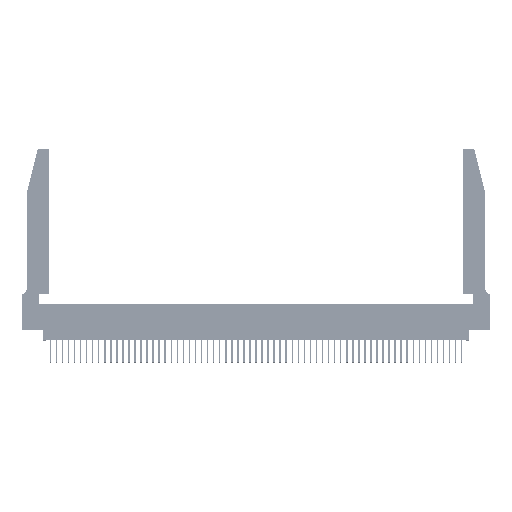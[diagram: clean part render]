
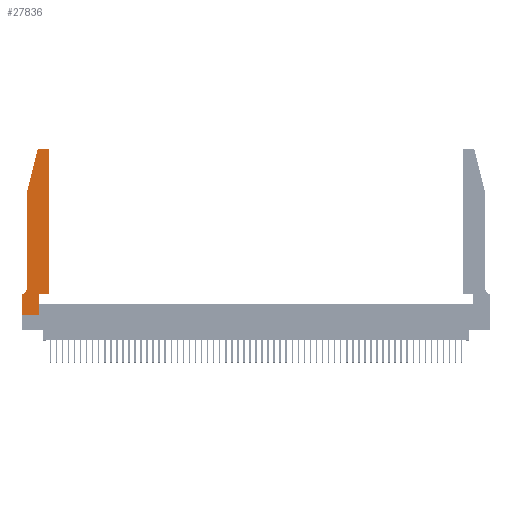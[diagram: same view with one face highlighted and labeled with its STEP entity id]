
A CAD part, top view. The second image highlights one B-rep face of the part: STEP entity #27836.
In plain terms, the highlighted planar face has unit normal (0, 0, 1).
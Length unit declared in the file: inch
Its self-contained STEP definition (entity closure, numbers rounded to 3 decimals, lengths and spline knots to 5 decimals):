
#403 = AXIS2_PLACEMENT_3D ( 'NONE', #30893, #5789, #18160 ) ;
#785 = EDGE_CURVE ( 'NONE', #35625, #1669, #9941, .T. ) ;
#947 = CARTESIAN_POINT ( 'NONE',  ( 0.284, 2.75, 0.37 ) ) ;
#1004 = ORIENTED_EDGE ( 'NONE', *, *, #785, .T. ) ;
#1669 = VERTEX_POINT ( 'NONE', #38193 ) ;
#1756 = VERTEX_POINT ( 'NONE', #46417 ) ;
#3053 = CARTESIAN_POINT ( 'NONE',  ( 0.4205, 2.72, 0.37 ) ) ;
#3824 = AXIS2_PLACEMENT_3D ( 'NONE', #3053, #15457, #7031 ) ;
#4704 = CARTESIAN_POINT ( 'NONE',  ( 0.4505, 0.35, 0.37 ) ) ;
#5002 = VERTEX_POINT ( 'NONE', #35126 ) ;
#5269 = DIRECTION ( 'NONE',  ( -1., 0., 0. ) ) ;
#5352 = ORIENTED_EDGE ( 'NONE', *, *, #52230, .T. ) ;
#5355 = VERTEX_POINT ( 'NONE', #29994 ) ;
#5673 = DIRECTION ( 'NONE',  ( -0.239, -0.971, 0. ) ) ;
#5789 = DIRECTION ( 'NONE',  ( 0., 0., 1. ) ) ;
#6862 = VECTOR ( 'NONE', #18560, 39.37008 ) ;
#7031 = DIRECTION ( 'NONE',  ( 1., 0., 0. ) ) ;
#7310 = CARTESIAN_POINT ( 'NONE',  ( 0.284, 2.72, 0.37 ) ) ;
#7510 = ORIENTED_EDGE ( 'NONE', *, *, #41520, .T. ) ;
#8234 = LINE ( 'NONE', #52009, #48363 ) ;
#9884 = VECTOR ( 'NONE', #24211, 39.37008 ) ;
#9941 = CIRCLE ( 'NONE', #3824, 0.03 ) ;
#10123 = EDGE_CURVE ( 'NONE', #1669, #36552, #8234, .T. ) ;
#11624 = DIRECTION ( 'NONE',  ( 1., 0., 0. ) ) ;
#12800 = VECTOR ( 'NONE', #5673, 39.37008 ) ;
#12887 = LINE ( 'NONE', #43791, #52960 ) ;
#13272 = VERTEX_POINT ( 'NONE', #48059 ) ;
#13618 = CARTESIAN_POINT ( 'NONE',  ( 0.0755, 2., 0.37 ) ) ;
#15457 = DIRECTION ( 'NONE',  ( 0., 0., 1. ) ) ;
#16917 = ORIENTED_EDGE ( 'NONE', *, *, #40889, .T. ) ;
#17618 = LINE ( 'NONE', #30756, #6862 ) ;
#18160 = DIRECTION ( 'NONE',  ( 1., 0., 0. ) ) ;
#18479 = CIRCLE ( 'NONE', #33254, 0.03 ) ;
#18560 = DIRECTION ( 'NONE',  ( 1., 0., 0. ) ) ;
#19590 = EDGE_CURVE ( 'NONE', #53398, #1756, #29552, .T. ) ;
#19633 = ORIENTED_EDGE ( 'NONE', *, *, #32566, .T. ) ;
#19774 = CARTESIAN_POINT ( 'NONE',  ( 0.25487, 2.72718, 0.37 ) ) ;
#20155 = CARTESIAN_POINT ( 'NONE',  ( 0.4505, 2.72, 0.37 ) ) ;
#21183 = DIRECTION ( 'NONE',  ( 1., 0., 0. ) ) ;
#22218 = DIRECTION ( 'NONE',  ( 0., -1., 0. ) ) ;
#22270 = AXIS2_PLACEMENT_3D ( 'NONE', #39279, #33523, #42101 ) ;
#24135 = ORIENTED_EDGE ( 'NONE', *, *, #49667, .T. ) ;
#24211 = DIRECTION ( 'NONE',  ( -1., 0., 0. ) ) ;
#24219 = EDGE_CURVE ( 'NONE', #32277, #42712, #30310, .T. ) ;
#25503 = EDGE_CURVE ( 'NONE', #33452, #5002, #47479, .T. ) ;
#26002 = VECTOR ( 'NONE', #43859, 39.37008 ) ;
#27297 = PLANE ( 'NONE',  #403 ) ;
#27557 = CARTESIAN_POINT ( 'NONE',  ( 0.4505, 0.35, 0.37 ) ) ;
#27836 = ADVANCED_FACE ( 'NONE', ( #40368 ), #27297, .T. ) ;
#29552 = LINE ( 'NONE', #48686, #12800 ) ;
#29994 = CARTESIAN_POINT ( 'NONE',  ( 0., 0.35, 0.37 ) ) ;
#30310 = LINE ( 'NONE', #4704, #47683 ) ;
#30756 = CARTESIAN_POINT ( 'NONE',  ( 0., 0., 0.37 ) ) ;
#30893 = CARTESIAN_POINT ( 'NONE',  ( 0., 0.35, 0.37 ) ) ;
#31427 = EDGE_CURVE ( 'NONE', #42712, #35625, #37385, .T. ) ;
#32277 = VERTEX_POINT ( 'NONE', #33971 ) ;
#32566 = EDGE_CURVE ( 'NONE', #36552, #53398, #18479, .T. ) ;
#33224 = ORIENTED_EDGE ( 'NONE', *, *, #19590, .T. ) ;
#33254 = AXIS2_PLACEMENT_3D ( 'NONE', #7310, #41540, #11624 ) ;
#33452 = VERTEX_POINT ( 'NONE', #46929 ) ;
#33523 = DIRECTION ( 'NONE',  ( 0., 0., -1. ) ) ;
#33971 = CARTESIAN_POINT ( 'NONE',  ( 0.2865, 0.35, 0.37 ) ) ;
#34423 = ORIENTED_EDGE ( 'NONE', *, *, #24219, .T. ) ;
#35126 = CARTESIAN_POINT ( 'NONE',  ( 0.0055, 0.35, 0.37 ) ) ;
#35601 = DIRECTION ( 'NONE',  ( 0., 1., 0. ) ) ;
#35625 = VERTEX_POINT ( 'NONE', #20155 ) ;
#36552 = VERTEX_POINT ( 'NONE', #947 ) ;
#37385 = LINE ( 'NONE', #27557, #26002 ) ;
#37498 = CARTESIAN_POINT ( 'NONE',  ( 0.0755, 0.35, 0.37 ) ) ;
#38193 = CARTESIAN_POINT ( 'NONE',  ( 0.4205, 2.75, 0.37 ) ) ;
#39279 = CARTESIAN_POINT ( 'NONE',  ( 0.0055, 0.42, 0.37 ) ) ;
#39545 = ORIENTED_EDGE ( 'NONE', *, *, #10123, .T. ) ;
#39900 = DIRECTION ( 'NONE',  ( 0., -1., 0. ) ) ;
#40368 = FACE_OUTER_BOUND ( 'NONE', #50018, .T. ) ;
#40889 = EDGE_CURVE ( 'NONE', #13272, #32277, #12887, .T. ) ;
#40894 = LINE ( 'NONE', #13618, #50931 ) ;
#41481 = ORIENTED_EDGE ( 'NONE', *, *, #31427, .T. ) ;
#41520 = EDGE_CURVE ( 'NONE', #1756, #33452, #40894, .T. ) ;
#41540 = DIRECTION ( 'NONE',  ( 0., 0., 1. ) ) ;
#41866 = CARTESIAN_POINT ( 'NONE',  ( 0., 0., 0.37 ) ) ;
#42101 = DIRECTION ( 'NONE',  ( -1., 0., 0. ) ) ;
#42712 = VERTEX_POINT ( 'NONE', #47709 ) ;
#43511 = VECTOR ( 'NONE', #39900, 39.37008 ) ;
#43791 = CARTESIAN_POINT ( 'NONE',  ( 0.2865, 0.35, 0.37 ) ) ;
#43859 = DIRECTION ( 'NONE',  ( 0., 1., 0. ) ) ;
#46417 = CARTESIAN_POINT ( 'NONE',  ( 0.0755, 2., 0.37 ) ) ;
#46929 = CARTESIAN_POINT ( 'NONE',  ( 0.0755, 0.42, 0.37 ) ) ;
#47384 = VERTEX_POINT ( 'NONE', #41866 ) ;
#47391 = LINE ( 'NONE', #37498, #9884 ) ;
#47479 = CIRCLE ( 'NONE', #22270, 0.07 ) ;
#47683 = VECTOR ( 'NONE', #21183, 39.37008 ) ;
#47709 = CARTESIAN_POINT ( 'NONE',  ( 0.4505, 0.35, 0.37 ) ) ;
#47957 = CARTESIAN_POINT ( 'NONE',  ( 0., 0., 0.37 ) ) ;
#48059 = CARTESIAN_POINT ( 'NONE',  ( 0.2865, 0., 0.37 ) ) ;
#48250 = EDGE_CURVE ( 'NONE', #5355, #47384, #50872, .T. ) ;
#48363 = VECTOR ( 'NONE', #5269, 39.37008 ) ;
#48686 = CARTESIAN_POINT ( 'NONE',  ( 0.0755, 2., 0.37 ) ) ;
#49667 = EDGE_CURVE ( 'NONE', #5002, #5355, #47391, .T. ) ;
#50018 = EDGE_LOOP ( 'NONE', ( #39545, #19633, #33224, #7510, #53065, #24135, #51752, #5352, #16917, #34423, #41481, #1004 ) ) ;
#50872 = LINE ( 'NONE', #47957, #43511 ) ;
#50931 = VECTOR ( 'NONE', #22218, 39.37008 ) ;
#51752 = ORIENTED_EDGE ( 'NONE', *, *, #48250, .T. ) ;
#52009 = CARTESIAN_POINT ( 'NONE',  ( 0.2605, 2.75, 0.37 ) ) ;
#52230 = EDGE_CURVE ( 'NONE', #47384, #13272, #17618, .T. ) ;
#52960 = VECTOR ( 'NONE', #35601, 39.37008 ) ;
#53065 = ORIENTED_EDGE ( 'NONE', *, *, #25503, .T. ) ;
#53398 = VERTEX_POINT ( 'NONE', #19774 ) ;
